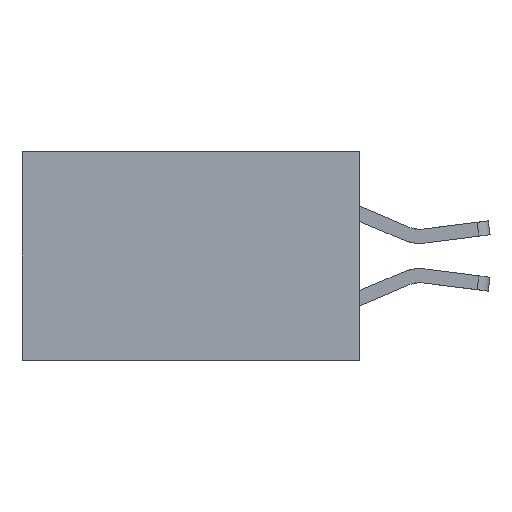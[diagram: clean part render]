
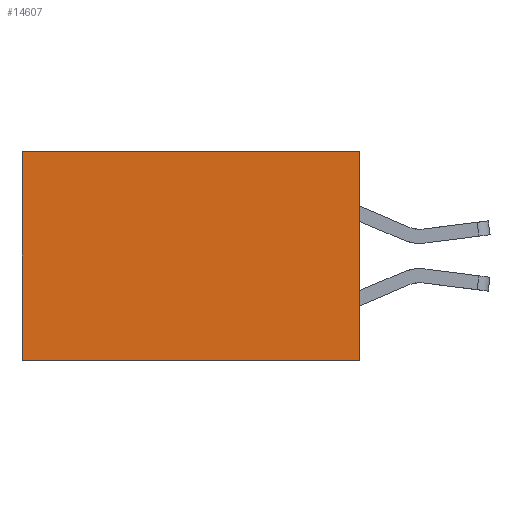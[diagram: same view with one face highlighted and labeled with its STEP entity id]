
A CAD part, left-side view. The second image highlights one B-rep face of the part: STEP entity #14607.
In plain terms, the highlighted planar face has unit normal (-1, 0, 0).
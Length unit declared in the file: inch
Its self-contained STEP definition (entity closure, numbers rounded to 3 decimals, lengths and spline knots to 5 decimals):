
#444 = DIRECTION ( 'NONE',  ( 0., 0., -1. ) ) ;
#486 = ORIENTED_EDGE ( 'NONE', *, *, #5135, .F. ) ;
#543 = ORIENTED_EDGE ( 'NONE', *, *, #11364, .T. ) ;
#1015 = CARTESIAN_POINT ( 'NONE',  ( 0.2875, 0., -0.37 ) ) ;
#1421 = DIRECTION ( 'NONE',  ( 0., 1., 0. ) ) ;
#1798 = CARTESIAN_POINT ( 'NONE',  ( 0.2875, 0., 0. ) ) ;
#2310 = CARTESIAN_POINT ( 'NONE',  ( 0.2875, 0.6, 0. ) ) ;
#2358 = VECTOR ( 'NONE', #1421, 39.37008 ) ;
#2995 = CARTESIAN_POINT ( 'NONE',  ( 0.2875, 0., 0. ) ) ;
#3386 = LINE ( 'NONE', #2310, #14198 ) ;
#4049 = VECTOR ( 'NONE', #14125, 39.37008 ) ;
#4200 = DIRECTION ( 'NONE',  ( 1., 0., 0. ) ) ;
#5135 = EDGE_CURVE ( 'NONE', #8856, #8094, #10687, .T. ) ;
#6404 = EDGE_CURVE ( 'NONE', #9202, #11223, #3386, .T. ) ;
#6460 = CARTESIAN_POINT ( 'NONE',  ( 0.2875, 0., 0. ) ) ;
#6647 = EDGE_CURVE ( 'NONE', #8094, #11223, #8591, .T. ) ;
#7761 = VECTOR ( 'NONE', #14249, 39.37008 ) ;
#8094 = VERTEX_POINT ( 'NONE', #14045 ) ;
#8591 = LINE ( 'NONE', #1015, #2358 ) ;
#8856 = VERTEX_POINT ( 'NONE', #1798 ) ;
#9202 = VERTEX_POINT ( 'NONE', #13740 ) ;
#9884 = PLANE ( 'NONE',  #12035 ) ;
#10089 = EDGE_LOOP ( 'NONE', ( #10559, #10603, #486, #543 ) ) ;
#10107 = LINE ( 'NONE', #6460, #4049 ) ;
#10559 = ORIENTED_EDGE ( 'NONE', *, *, #6404, .T. ) ;
#10603 = ORIENTED_EDGE ( 'NONE', *, *, #6647, .F. ) ;
#10687 = LINE ( 'NONE', #14019, #7761 ) ;
#11041 = FACE_OUTER_BOUND ( 'NONE', #10089, .T. ) ;
#11223 = VERTEX_POINT ( 'NONE', #11664 ) ;
#11364 = EDGE_CURVE ( 'NONE', #8856, #9202, #10107, .T. ) ;
#11664 = CARTESIAN_POINT ( 'NONE',  ( 0.2875, 0.6, -0.37 ) ) ;
#12017 = DIRECTION ( 'NONE',  ( 0., 0., -1. ) ) ;
#12035 = AXIS2_PLACEMENT_3D ( 'NONE', #2995, #4200, #12017 ) ;
#13740 = CARTESIAN_POINT ( 'NONE',  ( 0.2875, 0.6, 0. ) ) ;
#14019 = CARTESIAN_POINT ( 'NONE',  ( 0.2875, 0., 0. ) ) ;
#14045 = CARTESIAN_POINT ( 'NONE',  ( 0.2875, 0., -0.37 ) ) ;
#14125 = DIRECTION ( 'NONE',  ( 0., 1., 0. ) ) ;
#14198 = VECTOR ( 'NONE', #444, 39.37008 ) ;
#14249 = DIRECTION ( 'NONE',  ( 0., 0., -1. ) ) ;
#14607 = ADVANCED_FACE ( 'NONE', ( #11041 ), #9884, .F. ) ;
